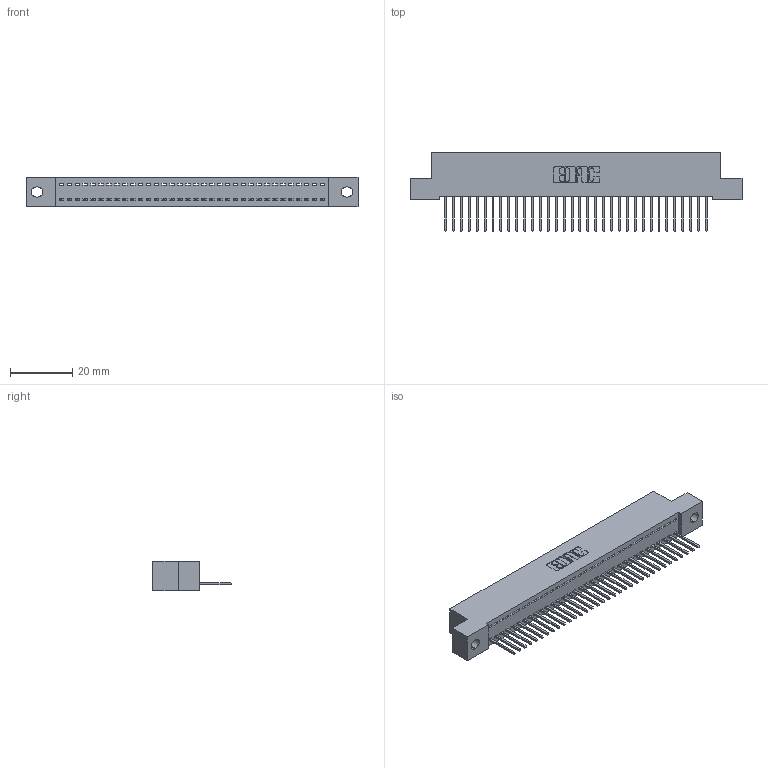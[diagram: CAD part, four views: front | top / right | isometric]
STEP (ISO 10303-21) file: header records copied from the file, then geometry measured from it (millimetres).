
FILE_DESCRIPTION (( 'STEP AP203' ), '1' );
FILE_NAME ('392-034-523-102.STEP', '2019-10-07T15:40:20', ( '' ), ( '' ), 'SwSTEP 2.0', 'SolidWorks 2016', '' );
FILE_SCHEMA (( 'CONFIG_CONTROL_DESIGN' ));
Length unit declared in the file: inch
Products named in the file (3): 345-292-001_345-293-123; 392-034-523-102; 342 Part_.128 Slot
Assembly tree (35 placements, depth 2):
  392-034-523-102
    342 Part_.128 Slot
    345-292-001_345-293-123  x34
Bounding box: 106.68 x 25.15 x 9.4 mm (x, y, z)
Volume: 9258.9 mm3; surface area: 13239 mm2
Topology: 35 solids, 35 shells, 2086 faces, 6295 edges, 4150 vertices
Faces by surface type: plane 1498, cylinder 588
Entity records: 21841 total; most frequent: CARTESIAN_POINT 3776, ORIENTED_EDGE 3746, DIRECTION 3201, EDGE_CURVE 1873, LINE 1745, VECTOR 1745, VERTEX_POINT 1246, AXIS2_PLACEMENT_3D 728
